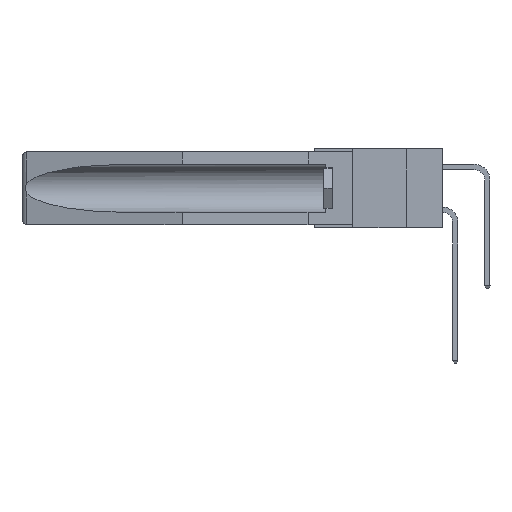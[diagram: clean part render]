
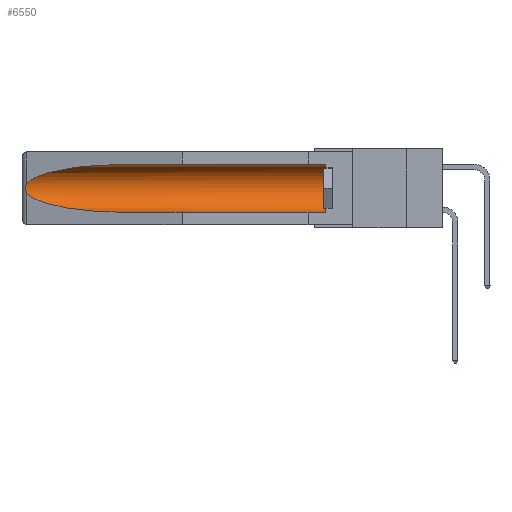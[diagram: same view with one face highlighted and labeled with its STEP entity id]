
A CAD part, left-side view. The second image highlights one B-rep face of the part: STEP entity #6550.
In plain terms, the highlighted cylindrical face has radius 2.857 mm (diameter 5.715 mm), a partial arc.
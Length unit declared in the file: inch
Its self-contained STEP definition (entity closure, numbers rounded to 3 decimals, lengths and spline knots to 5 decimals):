
#202 = CARTESIAN_POINT ( 'NONE',  ( 0.155, 1.07973, -0.284 ) ) ;
#280 =( BOUNDED_CURVE ( )  B_SPLINE_CURVE ( 3, ( #2135, #8238, #9695, #11343 ),
 .UNSPECIFIED., .F., .F. ) 
 B_SPLINE_CURVE_WITH_KNOTS ( ( 4, 4 ),
 ( 4.71239, 6.08839 ),
 .UNSPECIFIED. ) 
 CURVE ( )  GEOMETRIC_REPRESENTATION_ITEM ( )  RATIONAL_B_SPLINE_CURVE ( ( 1., 0.848, 0.848, 1. ) ) 
 REPRESENTATION_ITEM ( '' )  );
#414 = DIRECTION ( 'NONE',  ( 0., 0., 1. ) ) ;
#1542 = VECTOR ( 'NONE', #13696, 39.37008 ) ;
#2051 = EDGE_CURVE ( 'NONE', #18590, #8033, #3186, .T. ) ;
#2135 = CARTESIAN_POINT ( 'NONE',  ( 0.155, 1.07973, -0.059 ) ) ;
#2262 = CARTESIAN_POINT ( 'NONE',  ( 0.26654, 1.53092, -0.15636 ) ) ;
#2503 = EDGE_CURVE ( 'NONE', #14185, #18590, #280, .T. ) ;
#2603 = CARTESIAN_POINT ( 'NONE',  ( 0.155, -0.30754, -0.1715 ) ) ;
#3158 = DIRECTION ( 'NONE',  ( 0., -1., 0. ) ) ;
#3186 = B_SPLINE_CURVE_WITH_KNOTS ( 'NONE', 3,
 ( #11342, #14417, #2262, #8494, #17542, #9876, #12918, #14348, #18916, #3880 ),
 .UNSPECIFIED., .F., .F.,
 ( 4, 2, 2, 2, 4 ),
 ( 0., 0.00029, 0.00058, 0.00087, 0.00117 ),
 .UNSPECIFIED. ) ;
#3234 = EDGE_CURVE ( 'NONE', #12004, #14185, #6704, .T. ) ;
#3682 = CARTESIAN_POINT ( 'NONE',  ( 0.26537, 1.52718, -0.19328 ) ) ;
#3822 = CARTESIAN_POINT ( 'NONE',  ( 0.21114, 1.30732, -0.284 ) ) ;
#3880 = CARTESIAN_POINT ( 'NONE',  ( 0.26537, 1.52718, -0.19328 ) ) ;
#4677 = DIRECTION ( 'NONE',  ( 0., 1., 0. ) ) ;
#4748 = CARTESIAN_POINT ( 'NONE',  ( 0.155, 0.126, -0.059 ) ) ;
#5260 = CARTESIAN_POINT ( 'NONE',  ( 0.155, 1.07973, -0.284 ) ) ;
#6154 = DIRECTION ( 'NONE',  ( 0., 0., 1. ) ) ;
#6550 = ADVANCED_FACE ( 'NONE', ( #12273 ), #18650, .F. ) ;
#6704 = LINE ( 'NONE', #18581, #1542 ) ;
#6751 = CARTESIAN_POINT ( 'NONE',  ( 0.26537, 1.52718, -0.14972 ) ) ;
#7326 = ORIENTED_EDGE ( 'NONE', *, *, #14367, .T. ) ;
#7442 = CARTESIAN_POINT ( 'NONE',  ( 0.155, 1.07973, -0.059 ) ) ;
#8033 = VERTEX_POINT ( 'NONE', #3682 ) ;
#8238 = CARTESIAN_POINT ( 'NONE',  ( 0.21114, 1.30732, -0.059 ) ) ;
#8494 = CARTESIAN_POINT ( 'NONE',  ( 0.2673, 1.5327, -0.16383 ) ) ;
#8793 = ORIENTED_EDGE ( 'NONE', *, *, #15309, .F. ) ;
#9695 = CARTESIAN_POINT ( 'NONE',  ( 0.25451, 1.48313, -0.09465 ) ) ;
#9876 = CARTESIAN_POINT ( 'NONE',  ( 0.2675, 1.53308, -0.17534 ) ) ;
#10180 = VERTEX_POINT ( 'NONE', #13215 ) ;
#10375 = AXIS2_PLACEMENT_3D ( 'NONE', #2603, #16129, #414 ) ;
#10996 = EDGE_CURVE ( 'NONE', #10180, #12004, #18914, .T. ) ;
#11081 = CARTESIAN_POINT ( 'NONE',  ( 0.25451, 1.48313, -0.24835 ) ) ;
#11342 = CARTESIAN_POINT ( 'NONE',  ( 0.26537, 1.52718, -0.14972 ) ) ;
#11343 = CARTESIAN_POINT ( 'NONE',  ( 0.26537, 1.52718, -0.14972 ) ) ;
#12004 = VERTEX_POINT ( 'NONE', #4748 ) ;
#12273 = FACE_OUTER_BOUND ( 'NONE', #16841, .T. ) ;
#12811 = ORIENTED_EDGE ( 'NONE', *, *, #3234, .T. ) ;
#12918 = CARTESIAN_POINT ( 'NONE',  ( 0.2673, 1.53269, -0.17917 ) ) ;
#13215 = CARTESIAN_POINT ( 'NONE',  ( 0.155, 0.126, -0.284 ) ) ;
#13696 = DIRECTION ( 'NONE',  ( 0., 1., 0. ) ) ;
#13785 = CARTESIAN_POINT ( 'NONE',  ( 0.155, -0.30754, -0.284 ) ) ;
#14185 = VERTEX_POINT ( 'NONE', #7442 ) ;
#14348 = CARTESIAN_POINT ( 'NONE',  ( 0.26655, 1.53094, -0.18657 ) ) ;
#14367 = EDGE_CURVE ( 'NONE', #8033, #18432, #17096, .T. ) ;
#14417 = CARTESIAN_POINT ( 'NONE',  ( 0.26597, 1.52961, -0.15275 ) ) ;
#14705 = AXIS2_PLACEMENT_3D ( 'NONE', #15037, #3158, #6154 ) ;
#15037 = CARTESIAN_POINT ( 'NONE',  ( 0.155, 0.126, -0.1715 ) ) ;
#15309 = EDGE_CURVE ( 'NONE', #10180, #18432, #16896, .T. ) ;
#15389 = ORIENTED_EDGE ( 'NONE', *, *, #10996, .T. ) ;
#15531 = CARTESIAN_POINT ( 'NONE',  ( 0.26537, 1.52718, -0.19328 ) ) ;
#15906 = ORIENTED_EDGE ( 'NONE', *, *, #2051, .T. ) ;
#16129 = DIRECTION ( 'NONE',  ( 0., 1., 0. ) ) ;
#16411 = VECTOR ( 'NONE', #4677, 39.37008 ) ;
#16841 = EDGE_LOOP ( 'NONE', ( #19003, #15906, #7326, #8793, #15389, #12811 ) ) ;
#16896 = LINE ( 'NONE', #13785, #16411 ) ;
#17096 =( BOUNDED_CURVE ( )  B_SPLINE_CURVE ( 3, ( #15531, #11081, #3822, #5260 ),
 .UNSPECIFIED., .F., .F. ) 
 B_SPLINE_CURVE_WITH_KNOTS ( ( 4, 4 ),
 ( 0.1948, 1.5708 ),
 .UNSPECIFIED. ) 
 CURVE ( )  GEOMETRIC_REPRESENTATION_ITEM ( )  RATIONAL_B_SPLINE_CURVE ( ( 1., 0.848, 0.848, 1. ) ) 
 REPRESENTATION_ITEM ( '' )  );
#17542 = CARTESIAN_POINT ( 'NONE',  ( 0.2675, 1.53308, -0.16763 ) ) ;
#18432 = VERTEX_POINT ( 'NONE', #202 ) ;
#18581 = CARTESIAN_POINT ( 'NONE',  ( 0.155, -0.30754, -0.059 ) ) ;
#18590 = VERTEX_POINT ( 'NONE', #6751 ) ;
#18650 = CYLINDRICAL_SURFACE ( 'NONE', #10375, 0.1125 ) ;
#18914 = CIRCLE ( 'NONE', #14705, 0.1125 ) ;
#18916 = CARTESIAN_POINT ( 'NONE',  ( 0.26597, 1.5296, -0.19026 ) ) ;
#19003 = ORIENTED_EDGE ( 'NONE', *, *, #2503, .T. ) ;
